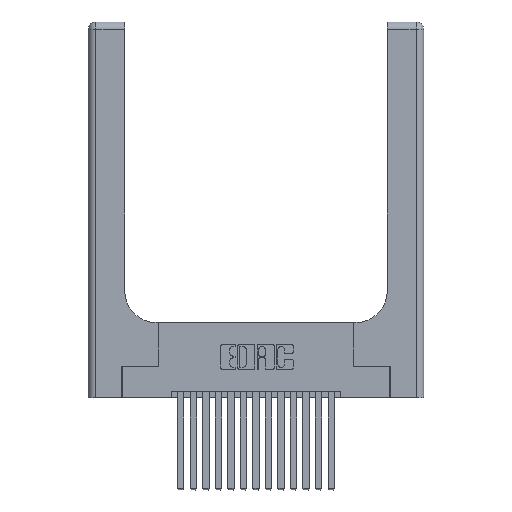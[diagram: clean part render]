
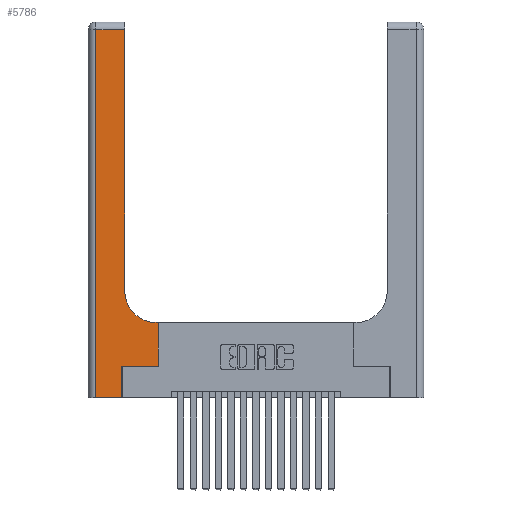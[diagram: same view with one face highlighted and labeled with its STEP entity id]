
A CAD part, top view. The second image highlights one B-rep face of the part: STEP entity #5786.
In plain terms, the highlighted planar face has unit normal (0, 0, 1).
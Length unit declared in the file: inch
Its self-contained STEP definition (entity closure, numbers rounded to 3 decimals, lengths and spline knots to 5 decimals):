
#31 = CARTESIAN_POINT ( 'NONE',  ( 0.2915, 0.85, 0.37 ) ) ;
#224 = VERTEX_POINT ( 'NONE', #4316 ) ;
#282 = ORIENTED_EDGE ( 'NONE', *, *, #15756, .T. ) ;
#283 = DIRECTION ( 'NONE',  ( 0., -1., 0. ) ) ;
#715 = ORIENTED_EDGE ( 'NONE', *, *, #1412, .T. ) ;
#757 = EDGE_CURVE ( 'NONE', #8652, #5394, #7413, .T. ) ;
#1412 = EDGE_CURVE ( 'NONE', #5761, #11745, #12022, .T. ) ;
#1740 = VECTOR ( 'NONE', #14632, 39.37008 ) ;
#1744 = ORIENTED_EDGE ( 'NONE', *, *, #8168, .T. ) ;
#2149 = DIRECTION ( 'NONE',  ( 0., 1., 0. ) ) ;
#2248 = CARTESIAN_POINT ( 'NONE',  ( 0.269, 0., 0.37 ) ) ;
#2544 = VERTEX_POINT ( 'NONE', #31 ) ;
#2784 = CARTESIAN_POINT ( 'NONE',  ( 0.269, 0., 0.37 ) ) ;
#2972 = FACE_OUTER_BOUND ( 'NONE', #6021, .T. ) ;
#3277 = CARTESIAN_POINT ( 'NONE',  ( 0.2915, 0.6, 0.37 ) ) ;
#3484 = ORIENTED_EDGE ( 'NONE', *, *, #7520, .T. ) ;
#3692 = DIRECTION ( 'NONE',  ( 0., 0., -1. ) ) ;
#3878 = LINE ( 'NONE', #6402, #18934 ) ;
#3895 = VERTEX_POINT ( 'NONE', #9314 ) ;
#4107 = EDGE_CURVE ( 'NONE', #14912, #2544, #14622, .T. ) ;
#4316 = CARTESIAN_POINT ( 'NONE',  ( 0.2915, 2.94, 0.37 ) ) ;
#4391 = LINE ( 'NONE', #8264, #7947 ) ;
#4560 = PLANE ( 'NONE',  #8753 ) ;
#4764 = DIRECTION ( 'NONE',  ( 1., 0., 0. ) ) ;
#5394 = VERTEX_POINT ( 'NONE', #2248 ) ;
#5761 = VERTEX_POINT ( 'NONE', #14799 ) ;
#5786 = ADVANCED_FACE ( 'NONE', ( #2972 ), #4560, .F. ) ;
#5902 = ORIENTED_EDGE ( 'NONE', *, *, #757, .T. ) ;
#6021 = EDGE_LOOP ( 'NONE', ( #282, #9910, #1744, #5902, #18496, #3484, #715, #13541, #11509 ) ) ;
#6095 = DIRECTION ( 'NONE',  ( 0., 0., -1. ) ) ;
#6402 = CARTESIAN_POINT ( 'NONE',  ( 0.06, 3., 0.37 ) ) ;
#6473 = VERTEX_POINT ( 'NONE', #7841 ) ;
#6849 = EDGE_CURVE ( 'NONE', #5394, #6473, #14081, .T. ) ;
#6947 = VECTOR ( 'NONE', #7145, 39.37008 ) ;
#6962 = VECTOR ( 'NONE', #4764, 39.37008 ) ;
#7145 = DIRECTION ( 'NONE',  ( 1., 0., 0. ) ) ;
#7413 = LINE ( 'NONE', #7916, #6947 ) ;
#7414 = DIRECTION ( 'NONE',  ( -1., 0., 0. ) ) ;
#7520 = EDGE_CURVE ( 'NONE', #6473, #5761, #14711, .T. ) ;
#7592 = AXIS2_PLACEMENT_3D ( 'NONE', #12642, #3692, #14046 ) ;
#7841 = CARTESIAN_POINT ( 'NONE',  ( 0.269, 0.25, 0.37 ) ) ;
#7916 = CARTESIAN_POINT ( 'NONE',  ( 0., 0., 0.37 ) ) ;
#7947 = VECTOR ( 'NONE', #2149, 39.37008 ) ;
#8092 = VECTOR ( 'NONE', #14356, 39.37008 ) ;
#8168 = EDGE_CURVE ( 'NONE', #3895, #8652, #3878, .T. ) ;
#8239 = LINE ( 'NONE', #3277, #12606 ) ;
#8264 = CARTESIAN_POINT ( 'NONE',  ( 0.2915, 3., 0.37 ) ) ;
#8652 = VERTEX_POINT ( 'NONE', #15155 ) ;
#8753 = AXIS2_PLACEMENT_3D ( 'NONE', #13440, #6095, #16301 ) ;
#9202 = CARTESIAN_POINT ( 'NONE',  ( 0.269, 0.25, 0.37 ) ) ;
#9314 = CARTESIAN_POINT ( 'NONE',  ( 0.06, 2.94, 0.37 ) ) ;
#9910 = ORIENTED_EDGE ( 'NONE', *, *, #10135, .T. ) ;
#10135 = EDGE_CURVE ( 'NONE', #224, #3895, #15097, .T. ) ;
#10182 = CARTESIAN_POINT ( 'NONE',  ( 0.5585, 0.6, 0.37 ) ) ;
#11509 = ORIENTED_EDGE ( 'NONE', *, *, #4107, .T. ) ;
#11745 = VERTEX_POINT ( 'NONE', #10182 ) ;
#11988 = EDGE_CURVE ( 'NONE', #11745, #14912, #8239, .T. ) ;
#12022 = LINE ( 'NONE', #14558, #8092 ) ;
#12606 = VECTOR ( 'NONE', #13671, 39.37008 ) ;
#12642 = CARTESIAN_POINT ( 'NONE',  ( 0.5415, 0.85, 0.37 ) ) ;
#13440 = CARTESIAN_POINT ( 'NONE',  ( 0., 3., 0.37 ) ) ;
#13541 = ORIENTED_EDGE ( 'NONE', *, *, #11988, .T. ) ;
#13671 = DIRECTION ( 'NONE',  ( -1., 0., 0. ) ) ;
#14046 = DIRECTION ( 'NONE',  ( 1., 0., 0. ) ) ;
#14081 = LINE ( 'NONE', #2784, #1740 ) ;
#14356 = DIRECTION ( 'NONE',  ( 0., 1., 0. ) ) ;
#14558 = CARTESIAN_POINT ( 'NONE',  ( 0.5585, 0.25, 0.37 ) ) ;
#14622 = CIRCLE ( 'NONE', #7592, 0.25 ) ;
#14632 = DIRECTION ( 'NONE',  ( 0., 1., 0. ) ) ;
#14647 = VECTOR ( 'NONE', #7414, 39.37008 ) ;
#14711 = LINE ( 'NONE', #9202, #6962 ) ;
#14799 = CARTESIAN_POINT ( 'NONE',  ( 0.5585, 0.25, 0.37 ) ) ;
#14912 = VERTEX_POINT ( 'NONE', #14923 ) ;
#14923 = CARTESIAN_POINT ( 'NONE',  ( 0.5415, 0.6, 0.37 ) ) ;
#15097 = LINE ( 'NONE', #18890, #14647 ) ;
#15155 = CARTESIAN_POINT ( 'NONE',  ( 0.06, 0., 0.37 ) ) ;
#15756 = EDGE_CURVE ( 'NONE', #2544, #224, #4391, .T. ) ;
#16301 = DIRECTION ( 'NONE',  ( -1., 0., 0. ) ) ;
#18496 = ORIENTED_EDGE ( 'NONE', *, *, #6849, .T. ) ;
#18890 = CARTESIAN_POINT ( 'NONE',  ( 0., 2.94, 0.37 ) ) ;
#18934 = VECTOR ( 'NONE', #283, 39.37008 ) ;
